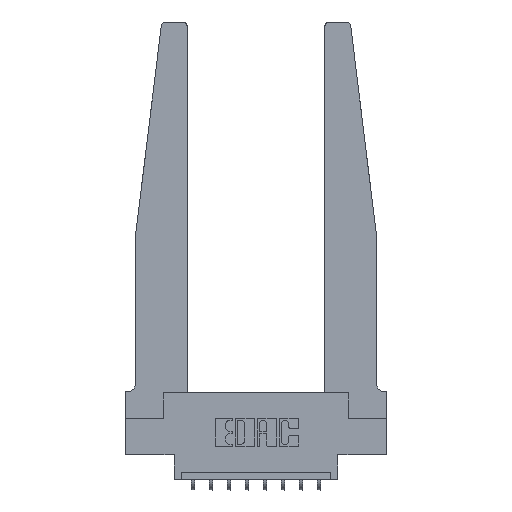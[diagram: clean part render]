
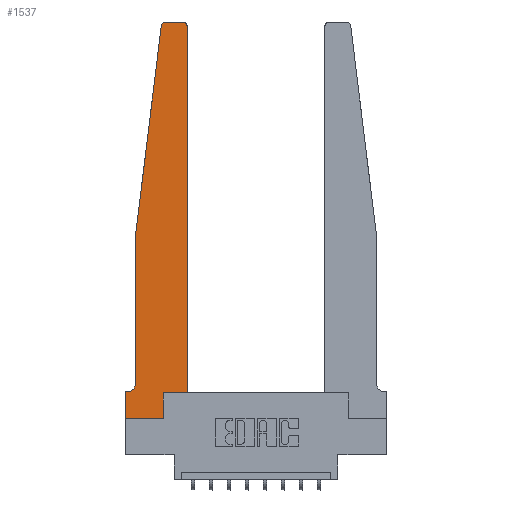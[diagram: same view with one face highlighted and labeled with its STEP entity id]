
A CAD part, top view. The second image highlights one B-rep face of the part: STEP entity #1537.
In plain terms, the highlighted planar face has unit normal (0, 0, 1).
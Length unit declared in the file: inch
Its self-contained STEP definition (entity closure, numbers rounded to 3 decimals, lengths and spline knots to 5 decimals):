
#13 = EDGE_CURVE ( 'NONE', #3372, #10883, #10482, .T. ) ;
#47 = DIRECTION ( 'NONE',  ( -1., 0., 0. ) ) ;
#336 = DIRECTION ( 'NONE',  ( 1., 0., 0. ) ) ;
#459 = DIRECTION ( 'NONE',  ( 1., 0., 0. ) ) ;
#689 = DIRECTION ( 'NONE',  ( 1., 0., 0. ) ) ;
#748 = CARTESIAN_POINT ( 'NONE',  ( 0., 0.1875, 0.37 ) ) ;
#826 = EDGE_CURVE ( 'NONE', #4696, #6702, #4716, .T. ) ;
#884 = DIRECTION ( 'NONE',  ( 0., -1., 0. ) ) ;
#893 = DIRECTION ( 'NONE',  ( -1., 0., 0. ) ) ;
#1024 = ORIENTED_EDGE ( 'NONE', *, *, #4088, .T. ) ;
#1027 = CARTESIAN_POINT ( 'NONE',  ( 0., 0., 0.37 ) ) ;
#1150 = DIRECTION ( 'NONE',  ( 0., 0., 1. ) ) ;
#1226 = ORIENTED_EDGE ( 'NONE', *, *, #826, .T. ) ;
#1353 = CARTESIAN_POINT ( 'NONE',  ( 0.065, 0.1875, 0.37 ) ) ;
#1488 = CARTESIAN_POINT ( 'NONE',  ( 0., 0., 0.37 ) ) ;
#1537 = ADVANCED_FACE ( 'NONE', ( #2782 ), #11074, .T. ) ;
#1776 = LINE ( 'NONE', #5261, #6191 ) ;
#2145 = ORIENTED_EDGE ( 'NONE', *, *, #13444, .T. ) ;
#2230 = AXIS2_PLACEMENT_3D ( 'NONE', #10941, #12996, #336 ) ;
#2527 = AXIS2_PLACEMENT_3D ( 'NONE', #12992, #1150, #4775 ) ;
#2634 = DIRECTION ( 'NONE',  ( 0., 0., 1. ) ) ;
#2782 = FACE_OUTER_BOUND ( 'NONE', #4787, .T. ) ;
#2902 = CARTESIAN_POINT ( 'NONE',  ( 0.425, 0.18, 0.37 ) ) ;
#2951 = DIRECTION ( 'NONE',  ( 1., 0., 0. ) ) ;
#2956 = EDGE_CURVE ( 'NONE', #10883, #12010, #8642, .T. ) ;
#3071 = DIRECTION ( 'NONE',  ( 0., 1., 0. ) ) ;
#3103 = CARTESIAN_POINT ( 'NONE',  ( 0.065, 1.25, 0.37 ) ) ;
#3152 = ORIENTED_EDGE ( 'NONE', *, *, #10964, .T. ) ;
#3344 = CARTESIAN_POINT ( 'NONE',  ( 0.065, 0.2375, 0.37 ) ) ;
#3372 = VERTEX_POINT ( 'NONE', #6632 ) ;
#3479 = VECTOR ( 'NONE', #47, 39.37008 ) ;
#3677 = ORIENTED_EDGE ( 'NONE', *, *, #12730, .T. ) ;
#3741 = CIRCLE ( 'NONE', #2527, 0.03 ) ;
#3752 = CARTESIAN_POINT ( 'NONE',  ( 0.24675, 2.72367, 0.37 ) ) ;
#3877 = EDGE_CURVE ( 'NONE', #9253, #3372, #13818, .T. ) ;
#3886 = CARTESIAN_POINT ( 'NONE',  ( 0.2605, 0., 0.37 ) ) ;
#4088 = EDGE_CURVE ( 'NONE', #6531, #9253, #3741, .T. ) ;
#4462 = EDGE_CURVE ( 'NONE', #6702, #4727, #10538, .T. ) ;
#4623 = AXIS2_PLACEMENT_3D ( 'NONE', #7563, #2634, #689 ) ;
#4696 = VERTEX_POINT ( 'NONE', #3344 ) ;
#4716 = CIRCLE ( 'NONE', #12488, 0.05 ) ;
#4727 = VERTEX_POINT ( 'NONE', #748 ) ;
#4775 = DIRECTION ( 'NONE',  ( 1., 0., 0. ) ) ;
#4787 = EDGE_LOOP ( 'NONE', ( #13430, #6870, #5406, #3677, #1226, #5485, #14648, #3152, #5077, #10658, #2145, #1024 ) ) ;
#5010 = EDGE_CURVE ( 'NONE', #12638, #14927, #14628, .T. ) ;
#5077 = ORIENTED_EDGE ( 'NONE', *, *, #5010, .T. ) ;
#5261 = CARTESIAN_POINT ( 'NONE',  ( 0., 0., 0.37 ) ) ;
#5406 = ORIENTED_EDGE ( 'NONE', *, *, #2956, .T. ) ;
#5485 = ORIENTED_EDGE ( 'NONE', *, *, #4462, .T. ) ;
#5658 = CARTESIAN_POINT ( 'NONE',  ( 0.065, 1.25, 0.37 ) ) ;
#5767 = CARTESIAN_POINT ( 'NONE',  ( 0.25, 2.75, 0.37 ) ) ;
#6191 = VECTOR ( 'NONE', #13749, 39.37008 ) ;
#6286 = VECTOR ( 'NONE', #459, 39.37008 ) ;
#6357 = CARTESIAN_POINT ( 'NONE',  ( 0.015, 0.1875, 0.37 ) ) ;
#6531 = VERTEX_POINT ( 'NONE', #10340 ) ;
#6627 = CARTESIAN_POINT ( 'NONE',  ( 0.015, 0.2375, 0.37 ) ) ;
#6632 = CARTESIAN_POINT ( 'NONE',  ( 0.27653, 2.75, 0.37 ) ) ;
#6702 = VERTEX_POINT ( 'NONE', #6357 ) ;
#6870 = ORIENTED_EDGE ( 'NONE', *, *, #13, .T. ) ;
#7176 = DIRECTION ( 'NONE',  ( -1., 0., 0. ) ) ;
#7197 = VECTOR ( 'NONE', #9799, 39.37008 ) ;
#7438 = CARTESIAN_POINT ( 'NONE',  ( 0.2605, 0.18, 0.37 ) ) ;
#7563 = CARTESIAN_POINT ( 'NONE',  ( 0., 0.1875, 0.37 ) ) ;
#7677 = VERTEX_POINT ( 'NONE', #1027 ) ;
#8003 = VECTOR ( 'NONE', #3071, 39.37008 ) ;
#8412 = EDGE_CURVE ( 'NONE', #4727, #7677, #1776, .T. ) ;
#8642 = LINE ( 'NONE', #3103, #7197 ) ;
#8674 = VECTOR ( 'NONE', #7176, 39.37008 ) ;
#8722 = DIRECTION ( 'NONE',  ( 0., 1., 0. ) ) ;
#8936 = LINE ( 'NONE', #9870, #9437 ) ;
#9042 = CARTESIAN_POINT ( 'NONE',  ( 0.065, 1.25, 0.37 ) ) ;
#9253 = VERTEX_POINT ( 'NONE', #10523 ) ;
#9437 = VECTOR ( 'NONE', #2951, 39.37008 ) ;
#9799 = DIRECTION ( 'NONE',  ( -0.122, -0.992, 0. ) ) ;
#9870 = CARTESIAN_POINT ( 'NONE',  ( 0.425, 0.18, 0.37 ) ) ;
#9913 = CARTESIAN_POINT ( 'NONE',  ( 0.425, 0.18, 0.37 ) ) ;
#10340 = CARTESIAN_POINT ( 'NONE',  ( 0.425, 2.72, 0.37 ) ) ;
#10393 = EDGE_CURVE ( 'NONE', #14927, #12635, #8936, .T. ) ;
#10482 = CIRCLE ( 'NONE', #2230, 0.03 ) ;
#10523 = CARTESIAN_POINT ( 'NONE',  ( 0.395, 2.75, 0.37 ) ) ;
#10538 = LINE ( 'NONE', #1353, #8674 ) ;
#10658 = ORIENTED_EDGE ( 'NONE', *, *, #10393, .T. ) ;
#10883 = VERTEX_POINT ( 'NONE', #3752 ) ;
#10918 = LINE ( 'NONE', #9913, #8003 ) ;
#10941 = CARTESIAN_POINT ( 'NONE',  ( 0.27653, 2.72, 0.37 ) ) ;
#10964 = EDGE_CURVE ( 'NONE', #7677, #12638, #11655, .T. ) ;
#11074 = PLANE ( 'NONE',  #4623 ) ;
#11276 = DIRECTION ( 'NONE',  ( 0., 0., -1. ) ) ;
#11499 = CARTESIAN_POINT ( 'NONE',  ( 0.2605, 0.18, 0.37 ) ) ;
#11655 = LINE ( 'NONE', #1488, #6286 ) ;
#11682 = VECTOR ( 'NONE', #8722, 39.37008 ) ;
#12010 = VERTEX_POINT ( 'NONE', #5658 ) ;
#12488 = AXIS2_PLACEMENT_3D ( 'NONE', #6627, #11276, #893 ) ;
#12635 = VERTEX_POINT ( 'NONE', #2902 ) ;
#12638 = VERTEX_POINT ( 'NONE', #3886 ) ;
#12730 = EDGE_CURVE ( 'NONE', #12010, #4696, #14870, .T. ) ;
#12992 = CARTESIAN_POINT ( 'NONE',  ( 0.395, 2.72, 0.37 ) ) ;
#12996 = DIRECTION ( 'NONE',  ( 0., 0., 1. ) ) ;
#13338 = VECTOR ( 'NONE', #884, 39.37008 ) ;
#13430 = ORIENTED_EDGE ( 'NONE', *, *, #3877, .T. ) ;
#13444 = EDGE_CURVE ( 'NONE', #12635, #6531, #10918, .T. ) ;
#13749 = DIRECTION ( 'NONE',  ( 0., -1., 0. ) ) ;
#13818 = LINE ( 'NONE', #5767, #3479 ) ;
#14628 = LINE ( 'NONE', #7438, #11682 ) ;
#14648 = ORIENTED_EDGE ( 'NONE', *, *, #8412, .T. ) ;
#14870 = LINE ( 'NONE', #9042, #13338 ) ;
#14927 = VERTEX_POINT ( 'NONE', #11499 ) ;
